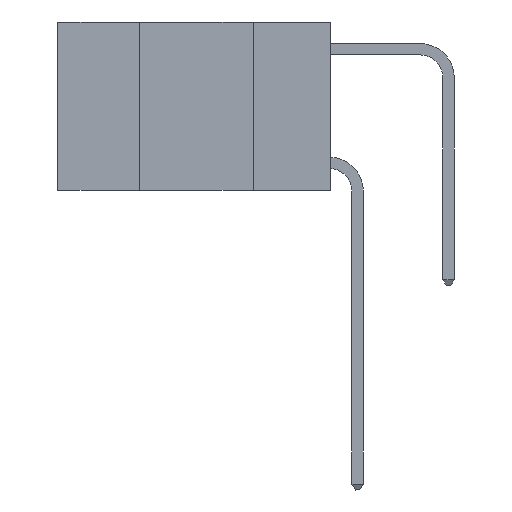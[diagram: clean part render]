
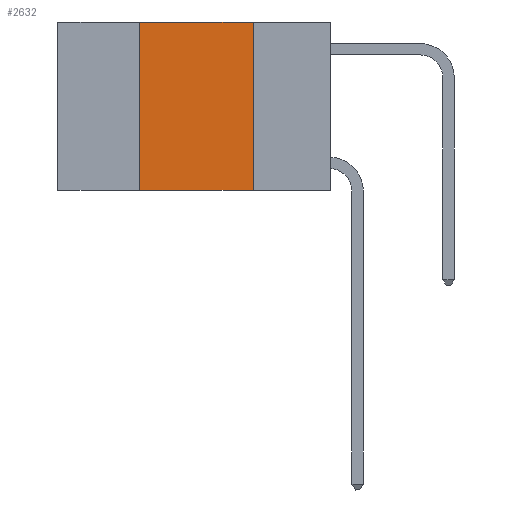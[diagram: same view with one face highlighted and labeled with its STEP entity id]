
A CAD part, left-side view. The second image highlights one B-rep face of the part: STEP entity #2632.
In plain terms, the highlighted planar face has unit normal (-1, 0, 0).
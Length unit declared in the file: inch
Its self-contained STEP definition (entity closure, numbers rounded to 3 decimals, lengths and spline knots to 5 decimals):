
#1127 = CARTESIAN_POINT ( 'NONE',  ( 0., 0.17, 0. ) ) ;
#1142 = LINE ( 'NONE', #1190, #8958 ) ;
#1190 = CARTESIAN_POINT ( 'NONE',  ( 0., 0.6, -0.37 ) ) ;
#1307 = DIRECTION ( 'NONE',  ( 0., 0., -1. ) ) ;
#1471 = VERTEX_POINT ( 'NONE', #1127 ) ;
#1681 = EDGE_CURVE ( 'NONE', #12626, #1471, #6942, .T. ) ;
#1816 = ORIENTED_EDGE ( 'NONE', *, *, #1681, .F. ) ;
#2632 = ADVANCED_FACE ( 'NONE', ( #11774 ), #9134, .F. ) ;
#3593 = VECTOR ( 'NONE', #8110, 39.37008 ) ;
#3753 = VECTOR ( 'NONE', #1307, 39.37008 ) ;
#6062 = VERTEX_POINT ( 'NONE', #11867 ) ;
#6392 = CARTESIAN_POINT ( 'NONE',  ( 0., 0.42, 0. ) ) ;
#6824 = AXIS2_PLACEMENT_3D ( 'NONE', #9036, #8974, #8971 ) ;
#6928 = CARTESIAN_POINT ( 'NONE',  ( 0., 0.42, -0.37 ) ) ;
#6942 = LINE ( 'NONE', #10905, #11664 ) ;
#7302 = ORIENTED_EDGE ( 'NONE', *, *, #9167, .F. ) ;
#7391 = DIRECTION ( 'NONE',  ( 0., -1., 0. ) ) ;
#7623 = ORIENTED_EDGE ( 'NONE', *, *, #12587, .T. ) ;
#7713 = VERTEX_POINT ( 'NONE', #6928 ) ;
#8110 = DIRECTION ( 'NONE',  ( 0., 0., 1. ) ) ;
#8958 = VECTOR ( 'NONE', #7391, 39.37008 ) ;
#8971 = DIRECTION ( 'NONE',  ( 0., 0., -1. ) ) ;
#8974 = DIRECTION ( 'NONE',  ( 1., 0., 0. ) ) ;
#9001 = LINE ( 'NONE', #10874, #3593 ) ;
#9036 = CARTESIAN_POINT ( 'NONE',  ( 0., 0.6, 0. ) ) ;
#9134 = PLANE ( 'NONE',  #6824 ) ;
#9141 = LINE ( 'NONE', #12137, #3753 ) ;
#9167 = EDGE_CURVE ( 'NONE', #7713, #12626, #9001, .T. ) ;
#9474 = EDGE_CURVE ( 'NONE', #1471, #6062, #9141, .T. ) ;
#10827 = DIRECTION ( 'NONE',  ( 0., -1., 0. ) ) ;
#10874 = CARTESIAN_POINT ( 'NONE',  ( 0., 0.42, 0. ) ) ;
#10905 = CARTESIAN_POINT ( 'NONE',  ( 0., 0.6, 0. ) ) ;
#11664 = VECTOR ( 'NONE', #10827, 39.37008 ) ;
#11740 = EDGE_LOOP ( 'NONE', ( #11981, #1816, #7302, #7623 ) ) ;
#11774 = FACE_OUTER_BOUND ( 'NONE', #11740, .T. ) ;
#11867 = CARTESIAN_POINT ( 'NONE',  ( 0., 0.17, -0.37 ) ) ;
#11981 = ORIENTED_EDGE ( 'NONE', *, *, #9474, .F. ) ;
#12137 = CARTESIAN_POINT ( 'NONE',  ( 0., 0.17, 0. ) ) ;
#12587 = EDGE_CURVE ( 'NONE', #7713, #6062, #1142, .T. ) ;
#12626 = VERTEX_POINT ( 'NONE', #6392 ) ;
